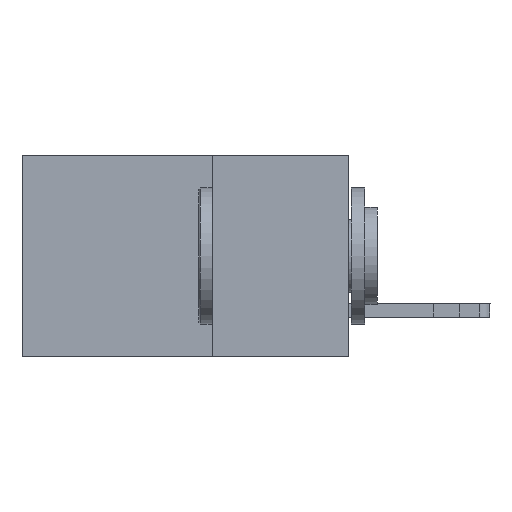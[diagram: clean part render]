
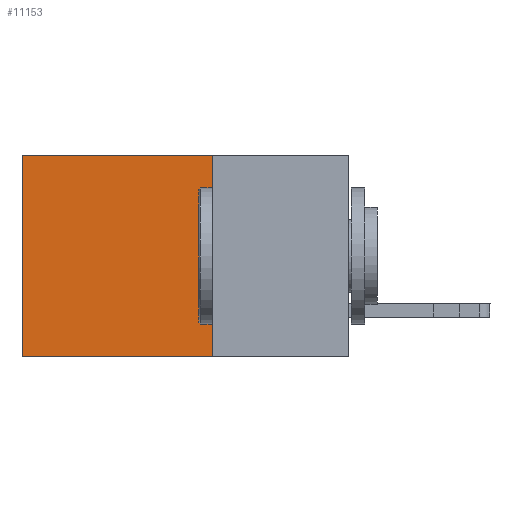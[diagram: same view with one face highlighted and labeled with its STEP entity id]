
A CAD part, left-side view. The second image highlights one B-rep face of the part: STEP entity #11153.
In plain terms, the highlighted planar face has unit normal (-1, 0, 0).
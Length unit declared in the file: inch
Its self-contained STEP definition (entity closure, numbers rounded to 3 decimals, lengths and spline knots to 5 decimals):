
#354 = DIRECTION ( 'NONE',  ( 0., 1., 0. ) ) ;
#520 = LINE ( 'NONE', #9145, #705 ) ;
#696 = CARTESIAN_POINT ( 'NONE',  ( 0.2615, 0.25, 0. ) ) ;
#705 = VECTOR ( 'NONE', #10261, 39.37008 ) ;
#1034 = CARTESIAN_POINT ( 'NONE',  ( 0.2615, 0.6, 0. ) ) ;
#1037 = CARTESIAN_POINT ( 'NONE',  ( 0.2615, 0.6, -0.37 ) ) ;
#1536 = DIRECTION ( 'NONE',  ( 1., 0., 0. ) ) ;
#1575 = EDGE_CURVE ( 'NONE', #3807, #8282, #520, .T. ) ;
#2229 = CARTESIAN_POINT ( 'NONE',  ( 0.2615, 0.25, -0.37 ) ) ;
#3007 = ORIENTED_EDGE ( 'NONE', *, *, #1575, .F. ) ;
#3807 = VERTEX_POINT ( 'NONE', #696 ) ;
#5363 = EDGE_CURVE ( 'NONE', #8282, #7125, #9728, .T. ) ;
#5869 = CARTESIAN_POINT ( 'NONE',  ( 0.2615, 0.25, -0.37 ) ) ;
#6483 = DIRECTION ( 'NONE',  ( 0., 1., 0. ) ) ;
#6718 = LINE ( 'NONE', #11927, #9486 ) ;
#6739 = EDGE_LOOP ( 'NONE', ( #12943, #13208, #3007, #10516 ) ) ;
#7125 = VERTEX_POINT ( 'NONE', #11666 ) ;
#8282 = VERTEX_POINT ( 'NONE', #13342 ) ;
#8604 = AXIS2_PLACEMENT_3D ( 'NONE', #5869, #1536, #9034 ) ;
#9034 = DIRECTION ( 'NONE',  ( 0., 0., -1. ) ) ;
#9145 = CARTESIAN_POINT ( 'NONE',  ( 0.2615, 0.25, -0.37 ) ) ;
#9486 = VECTOR ( 'NONE', #354, 39.37008 ) ;
#9718 = VECTOR ( 'NONE', #12735, 39.37008 ) ;
#9728 = LINE ( 'NONE', #2229, #13047 ) ;
#10026 = VERTEX_POINT ( 'NONE', #1034 ) ;
#10261 = DIRECTION ( 'NONE',  ( 0., 0., -1. ) ) ;
#10516 = ORIENTED_EDGE ( 'NONE', *, *, #13130, .T. ) ;
#11153 = ADVANCED_FACE ( 'NONE', ( #12268 ), #13094, .F. ) ;
#11426 = EDGE_CURVE ( 'NONE', #10026, #7125, #12869, .T. ) ;
#11666 = CARTESIAN_POINT ( 'NONE',  ( 0.2615, 0.6, -0.37 ) ) ;
#11927 = CARTESIAN_POINT ( 'NONE',  ( 0.2615, 0.25, 0. ) ) ;
#12268 = FACE_OUTER_BOUND ( 'NONE', #6739, .T. ) ;
#12735 = DIRECTION ( 'NONE',  ( 0., 0., -1. ) ) ;
#12869 = LINE ( 'NONE', #1037, #9718 ) ;
#12943 = ORIENTED_EDGE ( 'NONE', *, *, #11426, .T. ) ;
#13047 = VECTOR ( 'NONE', #6483, 39.37008 ) ;
#13094 = PLANE ( 'NONE',  #8604 ) ;
#13130 = EDGE_CURVE ( 'NONE', #3807, #10026, #6718, .T. ) ;
#13208 = ORIENTED_EDGE ( 'NONE', *, *, #5363, .F. ) ;
#13342 = CARTESIAN_POINT ( 'NONE',  ( 0.2615, 0.25, -0.37 ) ) ;
